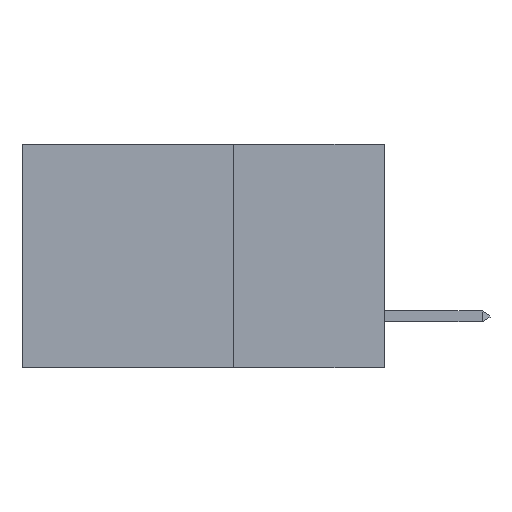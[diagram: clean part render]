
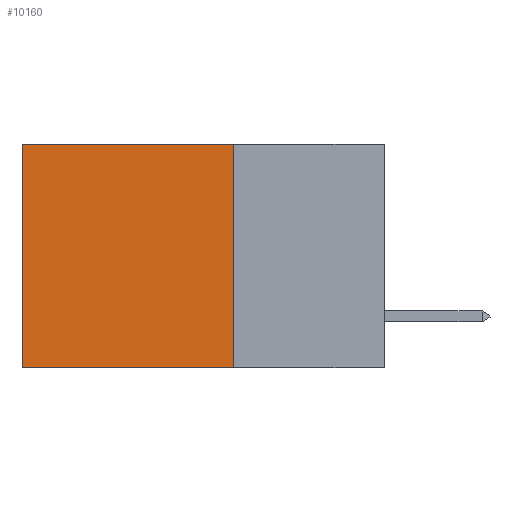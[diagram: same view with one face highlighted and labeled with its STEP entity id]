
A CAD part, left-side view. The second image highlights one B-rep face of the part: STEP entity #10160.
In plain terms, the highlighted planar face has unit normal (-1, 0, 0).
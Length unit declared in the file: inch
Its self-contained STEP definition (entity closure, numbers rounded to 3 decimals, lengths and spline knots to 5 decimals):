
#235 = LINE ( 'NONE', #9651, #7616 ) ;
#453 = VERTEX_POINT ( 'NONE', #14737 ) ;
#1098 = LINE ( 'NONE', #4680, #14695 ) ;
#2580 = VERTEX_POINT ( 'NONE', #9808 ) ;
#3464 = CARTESIAN_POINT ( 'NONE',  ( 0.2875, 0.25, 0. ) ) ;
#4173 = VERTEX_POINT ( 'NONE', #9347 ) ;
#4174 = CARTESIAN_POINT ( 'NONE',  ( 0.2875, 0.25, 0. ) ) ;
#4676 = EDGE_LOOP ( 'NONE', ( #7221, #13695, #13648, #12280 ) ) ;
#4680 = CARTESIAN_POINT ( 'NONE',  ( 0.2875, 0.25, 0. ) ) ;
#6984 = CARTESIAN_POINT ( 'NONE',  ( 0.2875, 0.6, 0. ) ) ;
#7181 = AXIS2_PLACEMENT_3D ( 'NONE', #3464, #7643, #16900 ) ;
#7221 = ORIENTED_EDGE ( 'NONE', *, *, #8350, .T. ) ;
#7616 = VECTOR ( 'NONE', #17497, 39.37008 ) ;
#7643 = DIRECTION ( 'NONE',  ( 1., 0., 0. ) ) ;
#8350 = EDGE_CURVE ( 'NONE', #17417, #2580, #13027, .T. ) ;
#9347 = CARTESIAN_POINT ( 'NONE',  ( 0.2875, 0.25, 0. ) ) ;
#9483 = VECTOR ( 'NONE', #15883, 39.37008 ) ;
#9651 = CARTESIAN_POINT ( 'NONE',  ( 0.2875, 0.25, -0.37 ) ) ;
#9808 = CARTESIAN_POINT ( 'NONE',  ( 0.2875, 0.6, -0.37 ) ) ;
#10160 = ADVANCED_FACE ( 'NONE', ( #14963 ), #15601, .F. ) ;
#10583 = VECTOR ( 'NONE', #16253, 39.37008 ) ;
#11708 = EDGE_CURVE ( 'NONE', #453, #2580, #235, .T. ) ;
#11996 = CARTESIAN_POINT ( 'NONE',  ( 0.2875, 0.6, 0. ) ) ;
#12280 = ORIENTED_EDGE ( 'NONE', *, *, #13182, .T. ) ;
#12872 = DIRECTION ( 'NONE',  ( 0., 1., 0. ) ) ;
#13027 = LINE ( 'NONE', #11996, #9483 ) ;
#13182 = EDGE_CURVE ( 'NONE', #4173, #17417, #1098, .T. ) ;
#13648 = ORIENTED_EDGE ( 'NONE', *, *, #15756, .F. ) ;
#13695 = ORIENTED_EDGE ( 'NONE', *, *, #11708, .F. ) ;
#14062 = LINE ( 'NONE', #4174, #10583 ) ;
#14695 = VECTOR ( 'NONE', #12872, 39.37008 ) ;
#14737 = CARTESIAN_POINT ( 'NONE',  ( 0.2875, 0.25, -0.37 ) ) ;
#14963 = FACE_OUTER_BOUND ( 'NONE', #4676, .T. ) ;
#15601 = PLANE ( 'NONE',  #7181 ) ;
#15756 = EDGE_CURVE ( 'NONE', #4173, #453, #14062, .T. ) ;
#15883 = DIRECTION ( 'NONE',  ( 0., 0., -1. ) ) ;
#16253 = DIRECTION ( 'NONE',  ( 0., 0., -1. ) ) ;
#16900 = DIRECTION ( 'NONE',  ( 0., 0., -1. ) ) ;
#17417 = VERTEX_POINT ( 'NONE', #6984 ) ;
#17497 = DIRECTION ( 'NONE',  ( 0., 1., 0. ) ) ;
